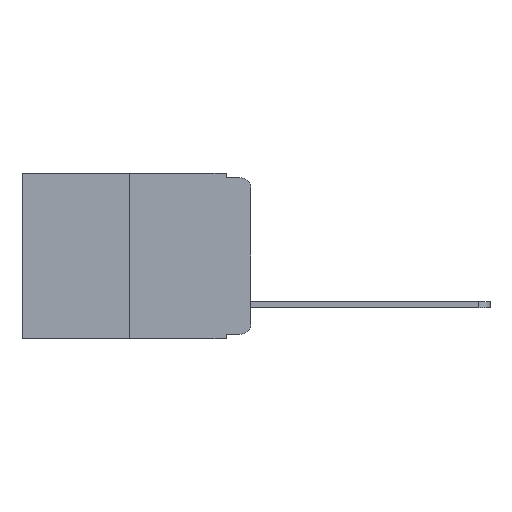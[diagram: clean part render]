
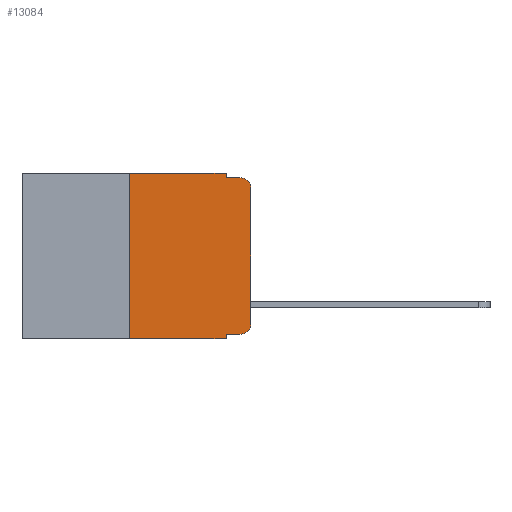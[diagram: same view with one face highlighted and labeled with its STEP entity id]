
A CAD part, left-side view. The second image highlights one B-rep face of the part: STEP entity #13084.
In plain terms, the highlighted planar face has unit normal (-1, 0, 0).
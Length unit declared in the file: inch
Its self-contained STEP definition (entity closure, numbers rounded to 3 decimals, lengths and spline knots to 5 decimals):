
#142 = LINE ( 'NONE', #10836, #4989 ) ;
#429 = ORIENTED_EDGE ( 'NONE', *, *, #12220, .F. ) ;
#526 = LINE ( 'NONE', #12039, #5361 ) ;
#622 = CARTESIAN_POINT ( 'NONE',  ( 0., 0.25, 0. ) ) ;
#752 = VERTEX_POINT ( 'NONE', #5829 ) ;
#835 = ORIENTED_EDGE ( 'NONE', *, *, #8484, .T. ) ;
#878 = EDGE_CURVE ( 'NONE', #10115, #7552, #2534, .T. ) ;
#972 = VECTOR ( 'NONE', #14188, 39.37008 ) ;
#1115 = VECTOR ( 'NONE', #8087, 39.37008 ) ;
#1309 = VERTEX_POINT ( 'NONE', #14578 ) ;
#1381 = VECTOR ( 'NONE', #11938, 39.37008 ) ;
#1960 = CARTESIAN_POINT ( 'NONE',  ( 0., 0.25, -0.343 ) ) ;
#2312 = CIRCLE ( 'NONE', #9438, 0.02 ) ;
#2407 = LINE ( 'NONE', #6796, #1115 ) ;
#2423 = DIRECTION ( 'NONE',  ( 0., 0., -1. ) ) ;
#2534 = LINE ( 'NONE', #4899, #13366 ) ;
#2684 = VERTEX_POINT ( 'NONE', #13911 ) ;
#2688 = ORIENTED_EDGE ( 'NONE', *, *, #11253, .T. ) ;
#3044 = DIRECTION ( 'NONE',  ( 0., 0., -1. ) ) ;
#3103 = CIRCLE ( 'NONE', #3956, 0.02 ) ;
#3664 = VECTOR ( 'NONE', #2423, 39.37008 ) ;
#3938 = CARTESIAN_POINT ( 'NONE',  ( 0., 0.02, -0.333 ) ) ;
#3956 = AXIS2_PLACEMENT_3D ( 'NONE', #4490, #5623, #5573 ) ;
#3962 = ORIENTED_EDGE ( 'NONE', *, *, #10480, .T. ) ;
#4490 = CARTESIAN_POINT ( 'NONE',  ( 0., 0.02, -0.313 ) ) ;
#4575 = LINE ( 'NONE', #10745, #1381 ) ;
#4837 = LINE ( 'NONE', #13658, #6879 ) ;
#4885 = VERTEX_POINT ( 'NONE', #13739 ) ;
#4899 = CARTESIAN_POINT ( 'NONE',  ( 0., 0.051, 0. ) ) ;
#4989 = VECTOR ( 'NONE', #6455, 39.37008 ) ;
#5094 = AXIS2_PLACEMENT_3D ( 'NONE', #11550, #10185, #3044 ) ;
#5173 = LINE ( 'NONE', #9557, #3664 ) ;
#5201 = CARTESIAN_POINT ( 'NONE',  ( 0., 0.051, -0.01 ) ) ;
#5361 = VECTOR ( 'NONE', #7597, 39.37008 ) ;
#5434 = VERTEX_POINT ( 'NONE', #1960 ) ;
#5573 = DIRECTION ( 'NONE',  ( 0., 0., -1. ) ) ;
#5623 = DIRECTION ( 'NONE',  ( -1., 0., 0. ) ) ;
#5829 = CARTESIAN_POINT ( 'NONE',  ( 0., 0.02, -0.01 ) ) ;
#6101 = VERTEX_POINT ( 'NONE', #3938 ) ;
#6202 = DIRECTION ( 'NONE',  ( 0., 0., -1. ) ) ;
#6455 = DIRECTION ( 'NONE',  ( 0., -1., 0. ) ) ;
#6500 = DIRECTION ( 'NONE',  ( 0., -1., 0. ) ) ;
#6520 = EDGE_LOOP ( 'NONE', ( #3962, #835, #10733, #11050, #429, #13058, #7349, #9351, #2688, #14642 ) ) ;
#6761 = LINE ( 'NONE', #9316, #972 ) ;
#6796 = CARTESIAN_POINT ( 'NONE',  ( 0., 0., 0. ) ) ;
#6879 = VECTOR ( 'NONE', #6500, 39.37008 ) ;
#7130 = EDGE_CURVE ( 'NONE', #6101, #2684, #3103, .T. ) ;
#7349 = ORIENTED_EDGE ( 'NONE', *, *, #15001, .T. ) ;
#7552 = VERTEX_POINT ( 'NONE', #5201 ) ;
#7597 = DIRECTION ( 'NONE',  ( 0., 0., 1. ) ) ;
#8087 = DIRECTION ( 'NONE',  ( 0., 0., 1. ) ) ;
#8484 = EDGE_CURVE ( 'NONE', #4885, #752, #2312, .T. ) ;
#8715 = DIRECTION ( 'NONE',  ( -1., 0., 0. ) ) ;
#8968 = PLANE ( 'NONE',  #5094 ) ;
#9316 = CARTESIAN_POINT ( 'NONE',  ( 0., 0.473, -0.343 ) ) ;
#9351 = ORIENTED_EDGE ( 'NONE', *, *, #12600, .F. ) ;
#9438 = AXIS2_PLACEMENT_3D ( 'NONE', #14635, #8715, #13290 ) ;
#9557 = CARTESIAN_POINT ( 'NONE',  ( 0., 0.051, 0. ) ) ;
#10058 = CARTESIAN_POINT ( 'NONE',  ( 0., 0.051, -0.343 ) ) ;
#10115 = VERTEX_POINT ( 'NONE', #14427 ) ;
#10185 = DIRECTION ( 'NONE',  ( 1., 0., 0. ) ) ;
#10480 = EDGE_CURVE ( 'NONE', #2684, #4885, #2407, .T. ) ;
#10733 = ORIENTED_EDGE ( 'NONE', *, *, #13954, .F. ) ;
#10745 = CARTESIAN_POINT ( 'NONE',  ( 0., 0.051, -0.01 ) ) ;
#10754 = FACE_OUTER_BOUND ( 'NONE', #6520, .T. ) ;
#10836 = CARTESIAN_POINT ( 'NONE',  ( 0., 0.473, 0. ) ) ;
#11050 = ORIENTED_EDGE ( 'NONE', *, *, #878, .F. ) ;
#11253 = EDGE_CURVE ( 'NONE', #1309, #6101, #4837, .T. ) ;
#11550 = CARTESIAN_POINT ( 'NONE',  ( 0., 0.473, 0. ) ) ;
#11938 = DIRECTION ( 'NONE',  ( 0., -1., 0. ) ) ;
#12039 = CARTESIAN_POINT ( 'NONE',  ( 0., 0.25, 0. ) ) ;
#12155 = EDGE_CURVE ( 'NONE', #5434, #14172, #526, .T. ) ;
#12220 = EDGE_CURVE ( 'NONE', #14172, #10115, #142, .T. ) ;
#12600 = EDGE_CURVE ( 'NONE', #1309, #13553, #5173, .T. ) ;
#13058 = ORIENTED_EDGE ( 'NONE', *, *, #12155, .F. ) ;
#13084 = ADVANCED_FACE ( 'NONE', ( #10754 ), #8968, .F. ) ;
#13290 = DIRECTION ( 'NONE',  ( 0., 0., -1. ) ) ;
#13366 = VECTOR ( 'NONE', #6202, 39.37008 ) ;
#13553 = VERTEX_POINT ( 'NONE', #10058 ) ;
#13658 = CARTESIAN_POINT ( 'NONE',  ( 0., 0.051, -0.333 ) ) ;
#13739 = CARTESIAN_POINT ( 'NONE',  ( 0., 0., -0.03 ) ) ;
#13911 = CARTESIAN_POINT ( 'NONE',  ( 0., 0., -0.313 ) ) ;
#13954 = EDGE_CURVE ( 'NONE', #7552, #752, #4575, .T. ) ;
#14172 = VERTEX_POINT ( 'NONE', #622 ) ;
#14188 = DIRECTION ( 'NONE',  ( 0., -1., 0. ) ) ;
#14427 = CARTESIAN_POINT ( 'NONE',  ( 0., 0.051, 0. ) ) ;
#14578 = CARTESIAN_POINT ( 'NONE',  ( 0., 0.051, -0.333 ) ) ;
#14635 = CARTESIAN_POINT ( 'NONE',  ( 0., 0.02, -0.03 ) ) ;
#14642 = ORIENTED_EDGE ( 'NONE', *, *, #7130, .T. ) ;
#15001 = EDGE_CURVE ( 'NONE', #5434, #13553, #6761, .T. ) ;
